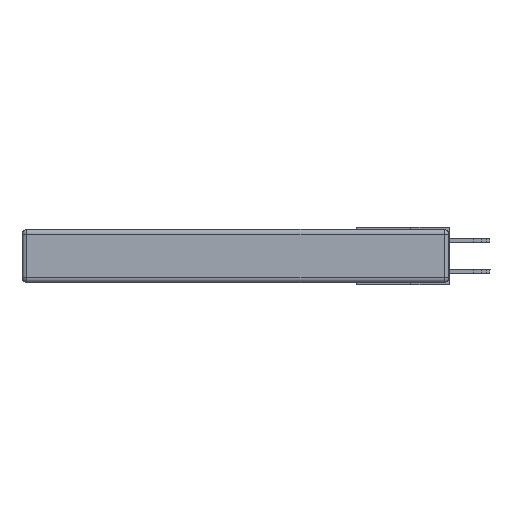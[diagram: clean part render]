
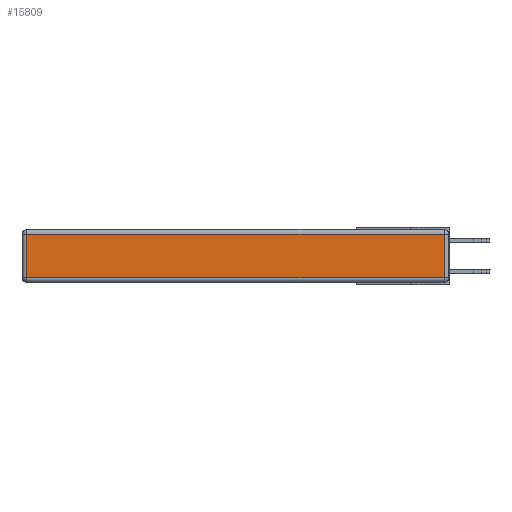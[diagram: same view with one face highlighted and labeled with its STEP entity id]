
A CAD part, left-side view. The second image highlights one B-rep face of the part: STEP entity #15809.
In plain terms, the highlighted planar face has unit normal (-1, 0, 0).
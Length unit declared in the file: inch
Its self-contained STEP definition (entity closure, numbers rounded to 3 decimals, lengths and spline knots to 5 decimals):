
#461 = VECTOR ( 'NONE', #2799, 39.37008 ) ;
#811 = DIRECTION ( 'NONE',  ( 0., 0., -1. ) ) ;
#1117 = CARTESIAN_POINT ( 'NONE',  ( 0., 2.75, -0.03 ) ) ;
#1485 = PLANE ( 'NONE',  #3518 ) ;
#2729 = LINE ( 'NONE', #1117, #17466 ) ;
#2784 = DIRECTION ( 'NONE',  ( -1., 0., 0. ) ) ;
#2799 = DIRECTION ( 'NONE',  ( 0., 0., 1. ) ) ;
#3518 = AXIS2_PLACEMENT_3D ( 'NONE', #4353, #2784, #19106 ) ;
#3566 = CARTESIAN_POINT ( 'NONE',  ( 0., 2.72, -0.313 ) ) ;
#3963 = ORIENTED_EDGE ( 'NONE', *, *, #15247, .T. ) ;
#4113 = CARTESIAN_POINT ( 'NONE',  ( 0., 0.03, -0.343 ) ) ;
#4353 = CARTESIAN_POINT ( 'NONE',  ( 0., 0., -0.343 ) ) ;
#6357 = CARTESIAN_POINT ( 'NONE',  ( 0., 0.03, -0.03 ) ) ;
#7446 = ORIENTED_EDGE ( 'NONE', *, *, #15561, .T. ) ;
#7812 = LINE ( 'NONE', #4113, #461 ) ;
#8195 = CARTESIAN_POINT ( 'NONE',  ( 0., 0.03, -0.313 ) ) ;
#9736 = VECTOR ( 'NONE', #18716, 39.37008 ) ;
#10235 = FACE_OUTER_BOUND ( 'NONE', #18101, .T. ) ;
#10251 = VECTOR ( 'NONE', #811, 39.37008 ) ;
#10295 = EDGE_CURVE ( 'NONE', #14287, #17657, #7812, .T. ) ;
#10815 = VERTEX_POINT ( 'NONE', #3566 ) ;
#10952 = LINE ( 'NONE', #13874, #10251 ) ;
#11471 = VERTEX_POINT ( 'NONE', #12099 ) ;
#11512 = ORIENTED_EDGE ( 'NONE', *, *, #17061, .T. ) ;
#12099 = CARTESIAN_POINT ( 'NONE',  ( 0., 2.72, -0.03 ) ) ;
#13874 = CARTESIAN_POINT ( 'NONE',  ( 0., 2.72, -0.343 ) ) ;
#14287 = VERTEX_POINT ( 'NONE', #8195 ) ;
#15247 = EDGE_CURVE ( 'NONE', #17657, #11471, #2729, .T. ) ;
#15553 = LINE ( 'NONE', #17217, #9736 ) ;
#15561 = EDGE_CURVE ( 'NONE', #11471, #10815, #10952, .T. ) ;
#15809 = ADVANCED_FACE ( 'NONE', ( #10235 ), #1485, .T. ) ;
#17061 = EDGE_CURVE ( 'NONE', #10815, #14287, #15553, .T. ) ;
#17217 = CARTESIAN_POINT ( 'NONE',  ( 0., 0., -0.313 ) ) ;
#17466 = VECTOR ( 'NONE', #18850, 39.37008 ) ;
#17657 = VERTEX_POINT ( 'NONE', #6357 ) ;
#18101 = EDGE_LOOP ( 'NONE', ( #11512, #19006, #3963, #7446 ) ) ;
#18716 = DIRECTION ( 'NONE',  ( 0., -1., 0. ) ) ;
#18850 = DIRECTION ( 'NONE',  ( 0., 1., 0. ) ) ;
#19006 = ORIENTED_EDGE ( 'NONE', *, *, #10295, .T. ) ;
#19106 = DIRECTION ( 'NONE',  ( 0., 0., 1. ) ) ;
